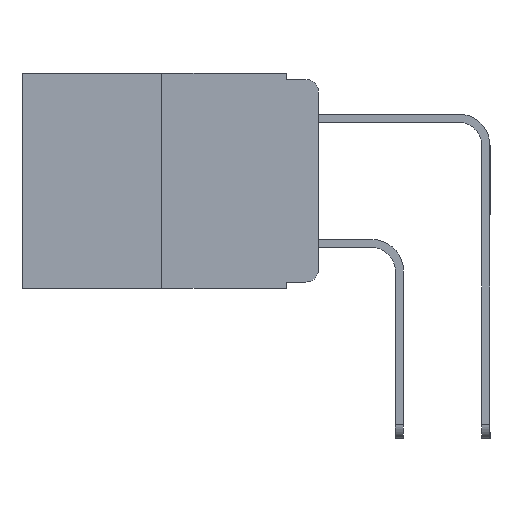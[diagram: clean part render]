
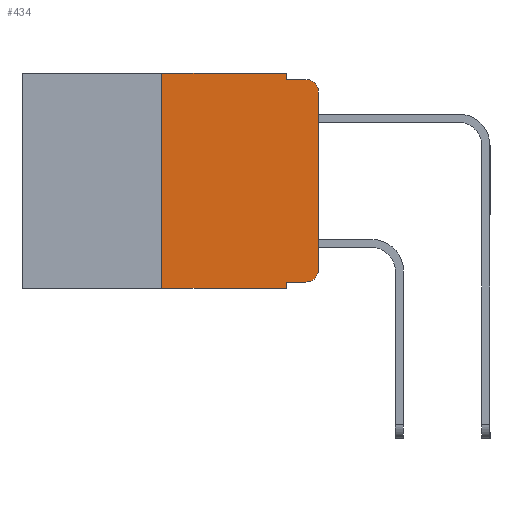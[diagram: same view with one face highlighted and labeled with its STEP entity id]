
A CAD part, left-side view. The second image highlights one B-rep face of the part: STEP entity #434.
In plain terms, the highlighted planar face has unit normal (-1, 0, 0).
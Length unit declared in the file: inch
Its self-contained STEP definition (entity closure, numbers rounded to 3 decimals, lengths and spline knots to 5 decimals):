
#238 = CARTESIAN_POINT ( 'NONE',  ( 0., 0.473, 0. ) ) ;
#434 = ADVANCED_FACE ( 'NONE', ( #17447 ), #8531, .F. ) ;
#738 = CARTESIAN_POINT ( 'NONE',  ( 0., 0.051, -0.343 ) ) ;
#755 = DIRECTION ( 'NONE',  ( 0., 0., -1. ) ) ;
#1038 = DIRECTION ( 'NONE',  ( -1., 0., 0. ) ) ;
#1056 = EDGE_LOOP ( 'NONE', ( #2408, #12842, #7314, #14158, #10500, #18674, #2451, #2424, #5710, #18909 ) ) ;
#1157 = VERTEX_POINT ( 'NONE', #20277 ) ;
#1300 = AXIS2_PLACEMENT_3D ( 'NONE', #238, #9209, #9953 ) ;
#2268 = CARTESIAN_POINT ( 'NONE',  ( 0., 0.02, -0.01 ) ) ;
#2408 = ORIENTED_EDGE ( 'NONE', *, *, #4706, .T. ) ;
#2424 = ORIENTED_EDGE ( 'NONE', *, *, #4145, .F. ) ;
#2451 = ORIENTED_EDGE ( 'NONE', *, *, #6742, .T. ) ;
#2937 = EDGE_CURVE ( 'NONE', #12272, #13895, #10717, .T. ) ;
#3090 = CARTESIAN_POINT ( 'NONE',  ( 0., 0.02, -0.03 ) ) ;
#3122 = VERTEX_POINT ( 'NONE', #738 ) ;
#3318 = AXIS2_PLACEMENT_3D ( 'NONE', #3090, #1038, #755 ) ;
#3449 = DIRECTION ( 'NONE',  ( -1., 0., 0. ) ) ;
#3670 = LINE ( 'NONE', #11970, #16538 ) ;
#4121 = DIRECTION ( 'NONE',  ( 0., 0., -1. ) ) ;
#4145 = EDGE_CURVE ( 'NONE', #1157, #3122, #15796, .T. ) ;
#4326 = LINE ( 'NONE', #9666, #21353 ) ;
#4706 = EDGE_CURVE ( 'NONE', #13895, #7442, #8229, .T. ) ;
#4743 = VECTOR ( 'NONE', #4121, 39.37008 ) ;
#5303 = EDGE_CURVE ( 'NONE', #17035, #6689, #18215, .T. ) ;
#5710 = ORIENTED_EDGE ( 'NONE', *, *, #19020, .T. ) ;
#5852 = EDGE_CURVE ( 'NONE', #7442, #8486, #21434, .T. ) ;
#5859 = DIRECTION ( 'NONE',  ( 0., 0., -1. ) ) ;
#6606 = CARTESIAN_POINT ( 'NONE',  ( 0., 0.473, 0. ) ) ;
#6689 = VERTEX_POINT ( 'NONE', #14679 ) ;
#6742 = EDGE_CURVE ( 'NONE', #16801, #3122, #18399, .T. ) ;
#6746 = DIRECTION ( 'NONE',  ( 0., -1., 0. ) ) ;
#7314 = ORIENTED_EDGE ( 'NONE', *, *, #15814, .F. ) ;
#7442 = VERTEX_POINT ( 'NONE', #13619 ) ;
#7709 = LINE ( 'NONE', #19206, #19236 ) ;
#7822 = DIRECTION ( 'NONE',  ( 0., 0., 1. ) ) ;
#7960 = CARTESIAN_POINT ( 'NONE',  ( 0., 0., 0. ) ) ;
#8125 = DIRECTION ( 'NONE',  ( 0., -1., 0. ) ) ;
#8229 = LINE ( 'NONE', #7960, #20726 ) ;
#8486 = VERTEX_POINT ( 'NONE', #2268 ) ;
#8531 = PLANE ( 'NONE',  #1300 ) ;
#9209 = DIRECTION ( 'NONE',  ( 1., 0., 0. ) ) ;
#9666 = CARTESIAN_POINT ( 'NONE',  ( 0., 0.051, -0.01 ) ) ;
#9953 = DIRECTION ( 'NONE',  ( 0., 0., -1. ) ) ;
#10500 = ORIENTED_EDGE ( 'NONE', *, *, #5303, .F. ) ;
#10717 = CIRCLE ( 'NONE', #15700, 0.02 ) ;
#10873 = DIRECTION ( 'NONE',  ( 0., 0., -1. ) ) ;
#11445 = DIRECTION ( 'NONE',  ( 0., -1., 0. ) ) ;
#11949 = VECTOR ( 'NONE', #5859, 39.37008 ) ;
#11970 = CARTESIAN_POINT ( 'NONE',  ( 0., 0.25, 0. ) ) ;
#12272 = VERTEX_POINT ( 'NONE', #19920 ) ;
#12842 = ORIENTED_EDGE ( 'NONE', *, *, #5852, .T. ) ;
#13619 = CARTESIAN_POINT ( 'NONE',  ( 0., 0., -0.03 ) ) ;
#13735 = LINE ( 'NONE', #14182, #4743 ) ;
#13895 = VERTEX_POINT ( 'NONE', #14436 ) ;
#13956 = VECTOR ( 'NONE', #6746, 39.37008 ) ;
#14158 = ORIENTED_EDGE ( 'NONE', *, *, #14729, .F. ) ;
#14182 = CARTESIAN_POINT ( 'NONE',  ( 0., 0.051, 0. ) ) ;
#14436 = CARTESIAN_POINT ( 'NONE',  ( 0., 0., -0.313 ) ) ;
#14640 = VECTOR ( 'NONE', #8125, 39.37008 ) ;
#14679 = CARTESIAN_POINT ( 'NONE',  ( 0., 0.051, 0. ) ) ;
#14729 = EDGE_CURVE ( 'NONE', #6689, #20208, #13735, .T. ) ;
#15380 = CARTESIAN_POINT ( 'NONE',  ( 0., 0.25, -0.343 ) ) ;
#15700 = AXIS2_PLACEMENT_3D ( 'NONE', #20429, #3449, #10873 ) ;
#15796 = LINE ( 'NONE', #18098, #11949 ) ;
#15814 = EDGE_CURVE ( 'NONE', #20208, #8486, #4326, .T. ) ;
#15978 = CARTESIAN_POINT ( 'NONE',  ( 0., 0.051, -0.01 ) ) ;
#16080 = DIRECTION ( 'NONE',  ( 0., -1., 0. ) ) ;
#16538 = VECTOR ( 'NONE', #18414, 39.37008 ) ;
#16801 = VERTEX_POINT ( 'NONE', #15380 ) ;
#17035 = VERTEX_POINT ( 'NONE', #17400 ) ;
#17400 = CARTESIAN_POINT ( 'NONE',  ( 0., 0.25, 0. ) ) ;
#17447 = FACE_OUTER_BOUND ( 'NONE', #1056, .T. ) ;
#17951 = EDGE_CURVE ( 'NONE', #16801, #17035, #3670, .T. ) ;
#18098 = CARTESIAN_POINT ( 'NONE',  ( 0., 0.051, 0. ) ) ;
#18215 = LINE ( 'NONE', #6606, #13956 ) ;
#18399 = LINE ( 'NONE', #19545, #14640 ) ;
#18414 = DIRECTION ( 'NONE',  ( 0., 0., 1. ) ) ;
#18674 = ORIENTED_EDGE ( 'NONE', *, *, #17951, .F. ) ;
#18909 = ORIENTED_EDGE ( 'NONE', *, *, #2937, .T. ) ;
#19020 = EDGE_CURVE ( 'NONE', #1157, #12272, #7709, .T. ) ;
#19206 = CARTESIAN_POINT ( 'NONE',  ( 0., 0.051, -0.333 ) ) ;
#19236 = VECTOR ( 'NONE', #16080, 39.37008 ) ;
#19545 = CARTESIAN_POINT ( 'NONE',  ( 0., 0.473, -0.343 ) ) ;
#19920 = CARTESIAN_POINT ( 'NONE',  ( 0., 0.02, -0.333 ) ) ;
#20208 = VERTEX_POINT ( 'NONE', #15978 ) ;
#20277 = CARTESIAN_POINT ( 'NONE',  ( 0., 0.051, -0.333 ) ) ;
#20429 = CARTESIAN_POINT ( 'NONE',  ( 0., 0.02, -0.313 ) ) ;
#20726 = VECTOR ( 'NONE', #7822, 39.37008 ) ;
#21353 = VECTOR ( 'NONE', #11445, 39.37008 ) ;
#21434 = CIRCLE ( 'NONE', #3318, 0.02 ) ;
